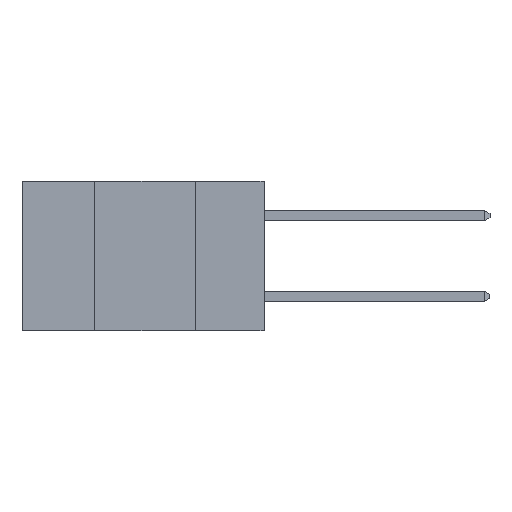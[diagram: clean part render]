
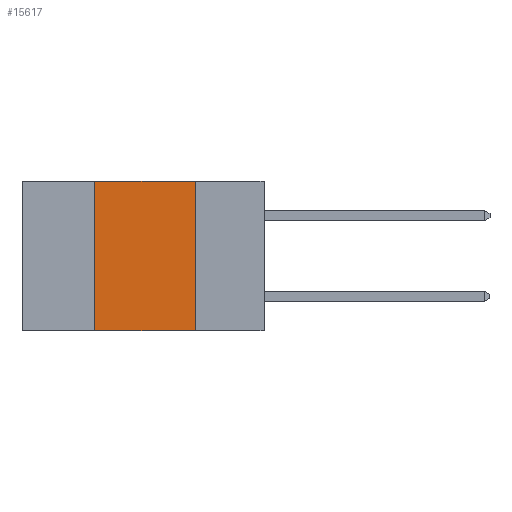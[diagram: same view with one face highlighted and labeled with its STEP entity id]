
A CAD part, left-side view. The second image highlights one B-rep face of the part: STEP entity #15617.
In plain terms, the highlighted planar face has unit normal (-1, 0, 0).
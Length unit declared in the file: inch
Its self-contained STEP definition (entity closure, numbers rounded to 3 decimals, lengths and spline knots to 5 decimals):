
#327 = ORIENTED_EDGE ( 'NONE', *, *, #15625, .F. ) ;
#563 = CARTESIAN_POINT ( 'NONE',  ( 0., 0.42, 0. ) ) ;
#804 = DIRECTION ( 'NONE',  ( 0., 0., -1. ) ) ;
#1103 = EDGE_CURVE ( 'NONE', #14075, #13493, #14010, .T. ) ;
#2150 = EDGE_CURVE ( 'NONE', #14075, #13249, #18626, .T. ) ;
#3176 = VECTOR ( 'NONE', #804, 39.37008 ) ;
#3297 = CARTESIAN_POINT ( 'NONE',  ( 0., 0.6, -0.37 ) ) ;
#6996 = DIRECTION ( 'NONE',  ( 0., 0., -1. ) ) ;
#8556 = CARTESIAN_POINT ( 'NONE',  ( 0., 0.17, 0. ) ) ;
#8625 = CARTESIAN_POINT ( 'NONE',  ( 0., 0.42, -0.37 ) ) ;
#8669 = DIRECTION ( 'NONE',  ( 0., -1., 0. ) ) ;
#8877 = CARTESIAN_POINT ( 'NONE',  ( 0., 0.42, 0. ) ) ;
#8927 = ORIENTED_EDGE ( 'NONE', *, *, #1103, .T. ) ;
#9548 = LINE ( 'NONE', #16401, #19225 ) ;
#9785 = VERTEX_POINT ( 'NONE', #10241 ) ;
#10241 = CARTESIAN_POINT ( 'NONE',  ( 0., 0.17, 0. ) ) ;
#10573 = DIRECTION ( 'NONE',  ( 0., -1., 0. ) ) ;
#12724 = EDGE_CURVE ( 'NONE', #13249, #9785, #9548, .T. ) ;
#13100 = CARTESIAN_POINT ( 'NONE',  ( 0., 0.6, 0. ) ) ;
#13249 = VERTEX_POINT ( 'NONE', #563 ) ;
#13402 = CARTESIAN_POINT ( 'NONE',  ( 0., 0.17, -0.37 ) ) ;
#13493 = VERTEX_POINT ( 'NONE', #13402 ) ;
#13501 = DIRECTION ( 'NONE',  ( 0., 0., 1. ) ) ;
#13531 = VECTOR ( 'NONE', #10573, 39.37008 ) ;
#13897 = ORIENTED_EDGE ( 'NONE', *, *, #2150, .F. ) ;
#14010 = LINE ( 'NONE', #3297, #13531 ) ;
#14075 = VERTEX_POINT ( 'NONE', #8625 ) ;
#14664 = PLANE ( 'NONE',  #19494 ) ;
#14698 = VECTOR ( 'NONE', #13501, 39.37008 ) ;
#15473 = FACE_OUTER_BOUND ( 'NONE', #18003, .T. ) ;
#15617 = ADVANCED_FACE ( 'NONE', ( #15473 ), #14664, .F. ) ;
#15625 = EDGE_CURVE ( 'NONE', #9785, #13493, #19342, .T. ) ;
#16227 = DIRECTION ( 'NONE',  ( 1., 0., 0. ) ) ;
#16401 = CARTESIAN_POINT ( 'NONE',  ( 0., 0.6, 0. ) ) ;
#18003 = EDGE_LOOP ( 'NONE', ( #327, #18452, #13897, #8927 ) ) ;
#18452 = ORIENTED_EDGE ( 'NONE', *, *, #12724, .F. ) ;
#18626 = LINE ( 'NONE', #8877, #14698 ) ;
#19225 = VECTOR ( 'NONE', #8669, 39.37008 ) ;
#19342 = LINE ( 'NONE', #8556, #3176 ) ;
#19494 = AXIS2_PLACEMENT_3D ( 'NONE', #13100, #16227, #6996 ) ;
